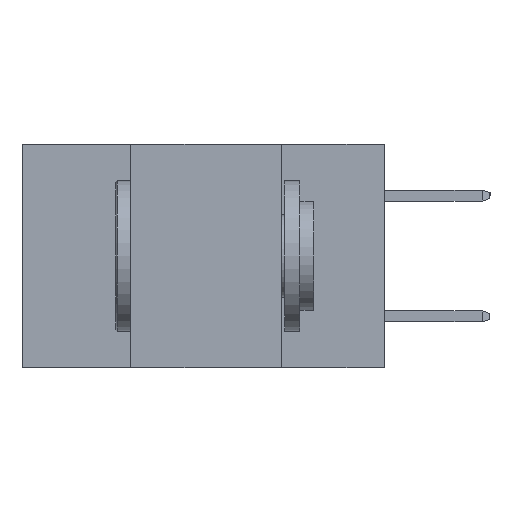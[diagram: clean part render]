
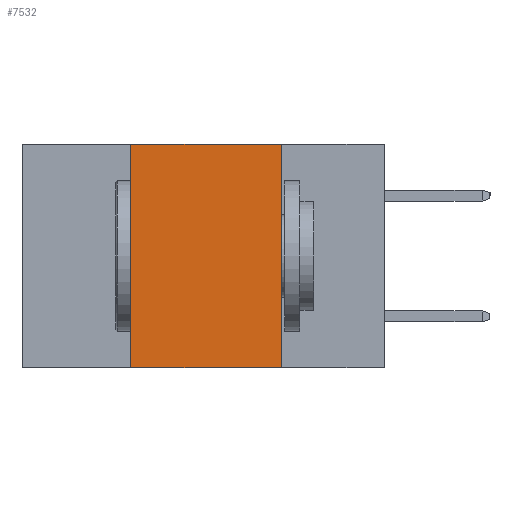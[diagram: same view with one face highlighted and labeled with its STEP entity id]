
A CAD part, left-side view. The second image highlights one B-rep face of the part: STEP entity #7532.
In plain terms, the highlighted planar face has unit normal (-1, 0, 0).
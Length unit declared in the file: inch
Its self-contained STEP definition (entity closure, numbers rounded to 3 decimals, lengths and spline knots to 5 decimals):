
#176 = CARTESIAN_POINT ( 'NONE',  ( 0., 0.6, 0. ) ) ;
#654 = VECTOR ( 'NONE', #1781, 39.37008 ) ;
#659 = EDGE_CURVE ( 'NONE', #7310, #5259, #12298, .T. ) ;
#1715 = DIRECTION ( 'NONE',  ( 0., 0., -1. ) ) ;
#1781 = DIRECTION ( 'NONE',  ( 0., 0., 1. ) ) ;
#1873 = VECTOR ( 'NONE', #8373, 39.37008 ) ;
#1980 = DIRECTION ( 'NONE',  ( 0., 0., -1. ) ) ;
#2599 = CARTESIAN_POINT ( 'NONE',  ( 0., 0.17, -0.37 ) ) ;
#2611 = EDGE_CURVE ( 'NONE', #2856, #5111, #7752, .T. ) ;
#2856 = VERTEX_POINT ( 'NONE', #12415 ) ;
#2961 = LINE ( 'NONE', #7903, #4307 ) ;
#3371 = CARTESIAN_POINT ( 'NONE',  ( 0., 0.42, -0.37 ) ) ;
#3535 = CARTESIAN_POINT ( 'NONE',  ( 0., 0.17, 0. ) ) ;
#3564 = PLANE ( 'NONE',  #4300 ) ;
#3923 = ORIENTED_EDGE ( 'NONE', *, *, #659, .T. ) ;
#4300 = AXIS2_PLACEMENT_3D ( 'NONE', #5810, #10722, #1715 ) ;
#4307 = VECTOR ( 'NONE', #1980, 39.37008 ) ;
#4359 = EDGE_CURVE ( 'NONE', #7310, #2856, #9999, .T. ) ;
#5066 = DIRECTION ( 'NONE',  ( 0., -1., 0. ) ) ;
#5111 = VERTEX_POINT ( 'NONE', #3535 ) ;
#5259 = VERTEX_POINT ( 'NONE', #2599 ) ;
#5472 = ORIENTED_EDGE ( 'NONE', *, *, #4359, .F. ) ;
#5810 = CARTESIAN_POINT ( 'NONE',  ( 0., 0.6, 0. ) ) ;
#6713 = FACE_OUTER_BOUND ( 'NONE', #11129, .T. ) ;
#6861 = ORIENTED_EDGE ( 'NONE', *, *, #2611, .F. ) ;
#7310 = VERTEX_POINT ( 'NONE', #3371 ) ;
#7508 = VECTOR ( 'NONE', #5066, 39.37008 ) ;
#7532 = ADVANCED_FACE ( 'NONE', ( #6713 ), #3564, .F. ) ;
#7752 = LINE ( 'NONE', #176, #7508 ) ;
#7903 = CARTESIAN_POINT ( 'NONE',  ( 0., 0.17, -0.37 ) ) ;
#7962 = CARTESIAN_POINT ( 'NONE',  ( 0., 0.42, -0.37 ) ) ;
#8300 = EDGE_CURVE ( 'NONE', #5111, #5259, #2961, .T. ) ;
#8373 = DIRECTION ( 'NONE',  ( 0., -1., 0. ) ) ;
#9696 = ORIENTED_EDGE ( 'NONE', *, *, #8300, .F. ) ;
#9999 = LINE ( 'NONE', #7962, #654 ) ;
#10722 = DIRECTION ( 'NONE',  ( 1., 0., 0. ) ) ;
#11129 = EDGE_LOOP ( 'NONE', ( #9696, #6861, #5472, #3923 ) ) ;
#11314 = CARTESIAN_POINT ( 'NONE',  ( 0., 0.6, -0.37 ) ) ;
#12298 = LINE ( 'NONE', #11314, #1873 ) ;
#12415 = CARTESIAN_POINT ( 'NONE',  ( 0., 0.42, 0. ) ) ;
